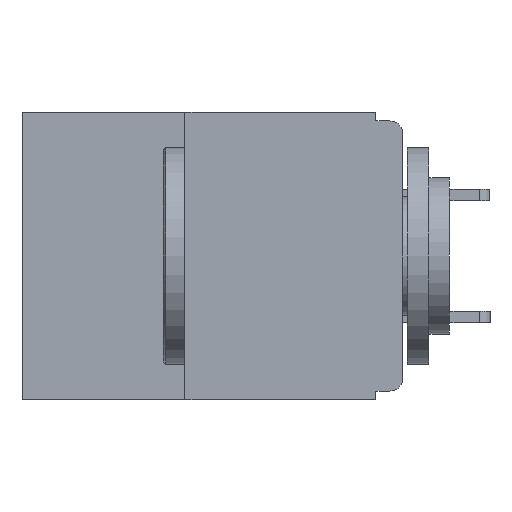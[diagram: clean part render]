
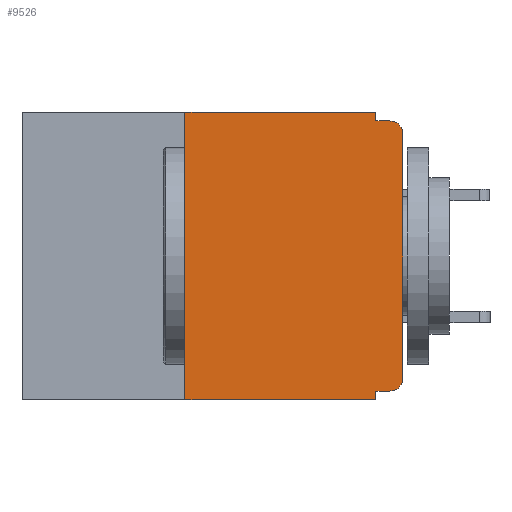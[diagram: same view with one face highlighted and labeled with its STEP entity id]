
A CAD part, left-side view. The second image highlights one B-rep face of the part: STEP entity #9526.
In plain terms, the highlighted planar face has unit normal (-1, 0, 0).
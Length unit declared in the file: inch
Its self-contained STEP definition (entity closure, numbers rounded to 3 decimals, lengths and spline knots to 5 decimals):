
#427 = VERTEX_POINT ( 'NONE', #8354 ) ;
#885 = EDGE_CURVE ( 'NONE', #6619, #9362, #9927, .T. ) ;
#936 = VECTOR ( 'NONE', #9631, 39.37008 ) ;
#1118 = DIRECTION ( 'NONE',  ( 0., 0., -1. ) ) ;
#1148 = DIRECTION ( 'NONE',  ( -1., 0., 0. ) ) ;
#1168 = CARTESIAN_POINT ( 'NONE',  ( 0., 0.015, -0.305 ) ) ;
#1274 = LINE ( 'NONE', #4947, #13484 ) ;
#1467 = VERTEX_POINT ( 'NONE', #5699 ) ;
#1793 = CARTESIAN_POINT ( 'NONE',  ( 0., 0.437, 0. ) ) ;
#1916 = ORIENTED_EDGE ( 'NONE', *, *, #6268, .F. ) ;
#2112 = LINE ( 'NONE', #4560, #14174 ) ;
#2174 = VERTEX_POINT ( 'NONE', #2377 ) ;
#2377 = CARTESIAN_POINT ( 'NONE',  ( 0., 0., -0.305 ) ) ;
#3232 = DIRECTION ( 'NONE',  ( 0., 0., -1. ) ) ;
#3371 = VERTEX_POINT ( 'NONE', #9343 ) ;
#3522 = CARTESIAN_POINT ( 'NONE',  ( 0., 0.25, 0. ) ) ;
#3871 = LINE ( 'NONE', #9747, #936 ) ;
#4246 = DIRECTION ( 'NONE',  ( 1., 0., 0. ) ) ;
#4250 = DIRECTION ( 'NONE',  ( 0., 0., 1. ) ) ;
#4560 = CARTESIAN_POINT ( 'NONE',  ( 0., 0., 0. ) ) ;
#4637 = EDGE_CURVE ( 'NONE', #11483, #6619, #3871, .T. ) ;
#4947 = CARTESIAN_POINT ( 'NONE',  ( 0., 0.031, 0. ) ) ;
#5131 = ORIENTED_EDGE ( 'NONE', *, *, #12482, .T. ) ;
#5305 = FACE_OUTER_BOUND ( 'NONE', #13313, .T. ) ;
#5321 = VERTEX_POINT ( 'NONE', #10399 ) ;
#5699 = CARTESIAN_POINT ( 'NONE',  ( 0., 0.031, 0. ) ) ;
#5718 = ORIENTED_EDGE ( 'NONE', *, *, #5842, .T. ) ;
#5842 = EDGE_CURVE ( 'NONE', #2174, #427, #2112, .T. ) ;
#5855 = ORIENTED_EDGE ( 'NONE', *, *, #7408, .T. ) ;
#5858 = DIRECTION ( 'NONE',  ( -1., 0., 0. ) ) ;
#5928 = ORIENTED_EDGE ( 'NONE', *, *, #15120, .F. ) ;
#6140 = ORIENTED_EDGE ( 'NONE', *, *, #12877, .F. ) ;
#6181 = DIRECTION ( 'NONE',  ( 0., -1., 0. ) ) ;
#6250 = CARTESIAN_POINT ( 'NONE',  ( 0., 0.031, -0.33 ) ) ;
#6268 = EDGE_CURVE ( 'NONE', #9979, #7249, #15202, .T. ) ;
#6393 = CARTESIAN_POINT ( 'NONE',  ( 0., 0.25, -0.33 ) ) ;
#6619 = VERTEX_POINT ( 'NONE', #13011 ) ;
#6684 = ORIENTED_EDGE ( 'NONE', *, *, #10763, .F. ) ;
#6861 = DIRECTION ( 'NONE',  ( 0., 0., 1. ) ) ;
#6941 = ORIENTED_EDGE ( 'NONE', *, *, #885, .F. ) ;
#7107 = CARTESIAN_POINT ( 'NONE',  ( 0., 0.25, -0.33 ) ) ;
#7249 = VERTEX_POINT ( 'NONE', #3522 ) ;
#7408 = EDGE_CURVE ( 'NONE', #11483, #2174, #14761, .T. ) ;
#7470 = VECTOR ( 'NONE', #9036, 39.37008 ) ;
#8134 = ORIENTED_EDGE ( 'NONE', *, *, #4637, .F. ) ;
#8239 = DIRECTION ( 'NONE',  ( 0., -1., 0. ) ) ;
#8354 = CARTESIAN_POINT ( 'NONE',  ( 0., 0., -0.025 ) ) ;
#9036 = DIRECTION ( 'NONE',  ( 0., -1., 0. ) ) ;
#9205 = AXIS2_PLACEMENT_3D ( 'NONE', #11305, #4246, #12460 ) ;
#9230 = VECTOR ( 'NONE', #6861, 39.37008 ) ;
#9343 = CARTESIAN_POINT ( 'NONE',  ( 0., 0.015, -0.01 ) ) ;
#9362 = VERTEX_POINT ( 'NONE', #6250 ) ;
#9526 = ADVANCED_FACE ( 'NONE', ( #5305 ), #11255, .F. ) ;
#9631 = DIRECTION ( 'NONE',  ( 0., 1., 0. ) ) ;
#9715 = DIRECTION ( 'NONE',  ( 0., 0., -1. ) ) ;
#9747 = CARTESIAN_POINT ( 'NONE',  ( 0., 0., -0.32 ) ) ;
#9889 = VECTOR ( 'NONE', #8239, 39.37008 ) ;
#9927 = LINE ( 'NONE', #13219, #10284 ) ;
#9972 = AXIS2_PLACEMENT_3D ( 'NONE', #1168, #1148, #1118 ) ;
#9979 = VERTEX_POINT ( 'NONE', #6393 ) ;
#10284 = VECTOR ( 'NONE', #3232, 39.37008 ) ;
#10399 = CARTESIAN_POINT ( 'NONE',  ( 0., 0.031, -0.01 ) ) ;
#10609 = LINE ( 'NONE', #1793, #7470 ) ;
#10681 = LINE ( 'NONE', #14254, #14661 ) ;
#10763 = EDGE_CURVE ( 'NONE', #5321, #3371, #10681, .T. ) ;
#11255 = PLANE ( 'NONE',  #9205 ) ;
#11305 = CARTESIAN_POINT ( 'NONE',  ( 0., 0.437, 0. ) ) ;
#11483 = VERTEX_POINT ( 'NONE', #13298 ) ;
#11771 = ORIENTED_EDGE ( 'NONE', *, *, #13091, .T. ) ;
#12460 = DIRECTION ( 'NONE',  ( 0., 0., -1. ) ) ;
#12482 = EDGE_CURVE ( 'NONE', #9979, #9362, #12566, .T. ) ;
#12566 = LINE ( 'NONE', #15031, #9889 ) ;
#12870 = CARTESIAN_POINT ( 'NONE',  ( 0., 0.015, -0.025 ) ) ;
#12877 = EDGE_CURVE ( 'NONE', #7249, #1467, #10609, .T. ) ;
#13011 = CARTESIAN_POINT ( 'NONE',  ( 0., 0.031, -0.32 ) ) ;
#13091 = EDGE_CURVE ( 'NONE', #427, #3371, #13739, .T. ) ;
#13219 = CARTESIAN_POINT ( 'NONE',  ( 0., 0.031, -0.33 ) ) ;
#13298 = CARTESIAN_POINT ( 'NONE',  ( 0., 0.015, -0.32 ) ) ;
#13313 = EDGE_LOOP ( 'NONE', ( #5718, #11771, #6684, #5928, #6140, #1916, #5131, #6941, #8134, #5855 ) ) ;
#13484 = VECTOR ( 'NONE', #9715, 39.37008 ) ;
#13581 = AXIS2_PLACEMENT_3D ( 'NONE', #12870, #5858, #13958 ) ;
#13739 = CIRCLE ( 'NONE', #13581, 0.015 ) ;
#13958 = DIRECTION ( 'NONE',  ( 0., 0., -1. ) ) ;
#14174 = VECTOR ( 'NONE', #4250, 39.37008 ) ;
#14254 = CARTESIAN_POINT ( 'NONE',  ( 0., 0., -0.01 ) ) ;
#14661 = VECTOR ( 'NONE', #6181, 39.37008 ) ;
#14761 = CIRCLE ( 'NONE', #9972, 0.015 ) ;
#15031 = CARTESIAN_POINT ( 'NONE',  ( 0., 0.437, -0.33 ) ) ;
#15120 = EDGE_CURVE ( 'NONE', #1467, #5321, #1274, .T. ) ;
#15202 = LINE ( 'NONE', #7107, #9230 ) ;
